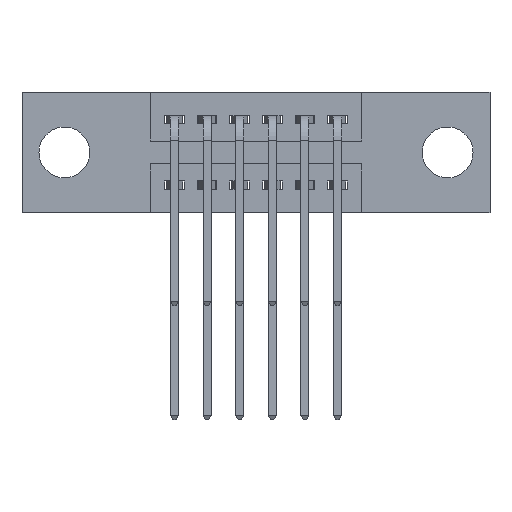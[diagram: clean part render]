
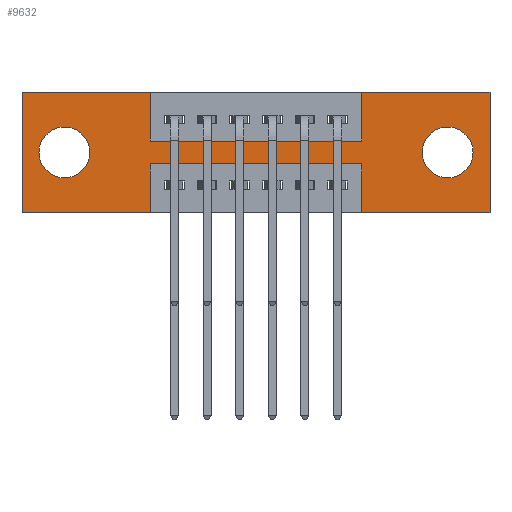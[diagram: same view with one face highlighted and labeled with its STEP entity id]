
A CAD part, front view. The second image highlights one B-rep face of the part: STEP entity #9632.
In plain terms, the highlighted planar face has unit normal (0, -1, 0).
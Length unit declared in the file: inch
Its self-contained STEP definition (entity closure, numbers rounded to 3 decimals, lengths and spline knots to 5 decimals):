
#202 = ORIENTED_EDGE ( 'NONE', *, *, #1817, .F. ) ;
#218 = EDGE_CURVE ( 'NONE', #5152, #11017, #5257, .T. ) ;
#248 = CARTESIAN_POINT ( 'NONE',  ( 1.435, 0., 0. ) ) ;
#366 = CARTESIAN_POINT ( 'NONE',  ( 1.0425, 0., 0. ) ) ;
#375 = ORIENTED_EDGE ( 'NONE', *, *, #869, .T. ) ;
#448 = ORIENTED_EDGE ( 'NONE', *, *, #2255, .F. ) ;
#457 = EDGE_LOOP ( 'NONE', ( #3153, #2119 ) ) ;
#676 = EDGE_CURVE ( 'NONE', #10058, #1149, #5128, .T. ) ;
#679 = CARTESIAN_POINT ( 'NONE',  ( 0.3925, 0., -0.15 ) ) ;
#805 = ORIENTED_EDGE ( 'NONE', *, *, #6886, .F. ) ;
#841 = ORIENTED_EDGE ( 'NONE', *, *, #6169, .F. ) ;
#858 = DIRECTION ( 'NONE',  ( -1., 0., 0. ) ) ;
#869 = EDGE_CURVE ( 'NONE', #1914, #2391, #6327, .T. ) ;
#880 = VECTOR ( 'NONE', #5306, 39.37008 ) ;
#924 = VERTEX_POINT ( 'NONE', #3868 ) ;
#1019 = LINE ( 'NONE', #8200, #11614 ) ;
#1138 = ORIENTED_EDGE ( 'NONE', *, *, #5997, .F. ) ;
#1149 = VERTEX_POINT ( 'NONE', #3234 ) ;
#1215 = ORIENTED_EDGE ( 'NONE', *, *, #7452, .F. ) ;
#1362 = CARTESIAN_POINT ( 'NONE',  ( 1.435, 0., 0. ) ) ;
#1496 = VERTEX_POINT ( 'NONE', #3971 ) ;
#1576 = ORIENTED_EDGE ( 'NONE', *, *, #4778, .F. ) ;
#1715 = CARTESIAN_POINT ( 'NONE',  ( 1.0425, 0., -0.22 ) ) ;
#1799 = VECTOR ( 'NONE', #5398, 39.37008 ) ;
#1817 = EDGE_CURVE ( 'NONE', #924, #9367, #1964, .T. ) ;
#1914 = VERTEX_POINT ( 'NONE', #6949 ) ;
#1964 = LINE ( 'NONE', #2258, #8264 ) ;
#2119 = ORIENTED_EDGE ( 'NONE', *, *, #8929, .T. ) ;
#2194 = CIRCLE ( 'NONE', #8778, 0.078 ) ;
#2255 = EDGE_CURVE ( 'NONE', #11017, #3963, #10328, .T. ) ;
#2258 = CARTESIAN_POINT ( 'NONE',  ( 0., 0., 0. ) ) ;
#2391 = VERTEX_POINT ( 'NONE', #8773 ) ;
#2502 = DIRECTION ( 'NONE',  ( 0., 0., -1. ) ) ;
#2565 = DIRECTION ( 'NONE',  ( 0., 0., -1. ) ) ;
#2607 = CARTESIAN_POINT ( 'NONE',  ( 1.0425, 0., 0. ) ) ;
#3078 = EDGE_LOOP ( 'NONE', ( #1576, #1138, #841, #6036, #448, #5516, #805, #4477, #9715, #202, #1215, #4601 ) ) ;
#3096 = DIRECTION ( 'NONE',  ( 0., 0., 1. ) ) ;
#3153 = ORIENTED_EDGE ( 'NONE', *, *, #5765, .T. ) ;
#3234 = CARTESIAN_POINT ( 'NONE',  ( 0., 0., -0.37 ) ) ;
#3313 = EDGE_LOOP ( 'NONE', ( #375, #4487 ) ) ;
#3424 = LINE ( 'NONE', #10508, #880 ) ;
#3464 = AXIS2_PLACEMENT_3D ( 'NONE', #5206, #7799, #11404 ) ;
#3525 = DIRECTION ( 'NONE',  ( 0., 0., 1. ) ) ;
#3554 = CARTESIAN_POINT ( 'NONE',  ( 0.13, 0., -0.107 ) ) ;
#3661 = VECTOR ( 'NONE', #7742, 39.37008 ) ;
#3772 = DIRECTION ( 'NONE',  ( 0., 0., 1. ) ) ;
#3849 = VECTOR ( 'NONE', #5325, 39.37008 ) ;
#3868 = CARTESIAN_POINT ( 'NONE',  ( 0., 0., 0. ) ) ;
#3963 = VERTEX_POINT ( 'NONE', #11116 ) ;
#3971 = CARTESIAN_POINT ( 'NONE',  ( 0.13, 0., -0.263 ) ) ;
#4007 = VECTOR ( 'NONE', #7783, 39.37008 ) ;
#4046 = VECTOR ( 'NONE', #4680, 39.37008 ) ;
#4062 = DIRECTION ( 'NONE',  ( 0., 0., 1. ) ) ;
#4194 = FACE_BOUND ( 'NONE', #457, .T. ) ;
#4234 = AXIS2_PLACEMENT_3D ( 'NONE', #6861, #5048, #3096 ) ;
#4254 = PLANE ( 'NONE',  #3464 ) ;
#4477 = ORIENTED_EDGE ( 'NONE', *, *, #9099, .F. ) ;
#4487 = ORIENTED_EDGE ( 'NONE', *, *, #6104, .T. ) ;
#4601 = ORIENTED_EDGE ( 'NONE', *, *, #676, .F. ) ;
#4642 = CARTESIAN_POINT ( 'NONE',  ( 1.305, 0., -0.185 ) ) ;
#4680 = DIRECTION ( 'NONE',  ( -1., 0., 0. ) ) ;
#4729 = DIRECTION ( 'NONE',  ( 0., 1., 0. ) ) ;
#4734 = LINE ( 'NONE', #5684, #4046 ) ;
#4778 = EDGE_CURVE ( 'NONE', #5113, #10058, #9640, .T. ) ;
#4889 = VECTOR ( 'NONE', #11262, 39.37008 ) ;
#5048 = DIRECTION ( 'NONE',  ( 0., 1., 0. ) ) ;
#5113 = VERTEX_POINT ( 'NONE', #7904 ) ;
#5128 = LINE ( 'NONE', #5892, #4007 ) ;
#5146 = CARTESIAN_POINT ( 'NONE',  ( 0.3925, 0., -0.37 ) ) ;
#5152 = VERTEX_POINT ( 'NONE', #2607 ) ;
#5206 = CARTESIAN_POINT ( 'NONE',  ( 0., 0., -0.37 ) ) ;
#5208 = VECTOR ( 'NONE', #4062, 39.37008 ) ;
#5257 = LINE ( 'NONE', #11345, #3661 ) ;
#5297 = DIRECTION ( 'NONE',  ( 0., 1., 0. ) ) ;
#5306 = DIRECTION ( 'NONE',  ( 0., 0., -1. ) ) ;
#5325 = DIRECTION ( 'NONE',  ( 1., 0., 0. ) ) ;
#5398 = DIRECTION ( 'NONE',  ( 0., 0., 1. ) ) ;
#5516 = ORIENTED_EDGE ( 'NONE', *, *, #218, .F. ) ;
#5606 = VERTEX_POINT ( 'NONE', #11378 ) ;
#5684 = CARTESIAN_POINT ( 'NONE',  ( 0., 0., -0.37 ) ) ;
#5765 = EDGE_CURVE ( 'NONE', #7993, #1496, #5954, .T. ) ;
#5892 = CARTESIAN_POINT ( 'NONE',  ( 0., 0., -0.37 ) ) ;
#5954 = CIRCLE ( 'NONE', #6139, 0.078 ) ;
#5997 = EDGE_CURVE ( 'NONE', #11311, #5113, #11640, .T. ) ;
#6036 = ORIENTED_EDGE ( 'NONE', *, *, #8811, .F. ) ;
#6104 = EDGE_CURVE ( 'NONE', #2391, #1914, #2194, .T. ) ;
#6139 = AXIS2_PLACEMENT_3D ( 'NONE', #9226, #4729, #3525 ) ;
#6144 = FACE_BOUND ( 'NONE', #3313, .T. ) ;
#6169 = EDGE_CURVE ( 'NONE', #8464, #11311, #1019, .T. ) ;
#6327 = CIRCLE ( 'NONE', #8397, 0.078 ) ;
#6491 = EDGE_CURVE ( 'NONE', #9367, #8373, #3424, .T. ) ;
#6861 = CARTESIAN_POINT ( 'NONE',  ( 0.13, 0., -0.185 ) ) ;
#6886 = EDGE_CURVE ( 'NONE', #5606, #5152, #9314, .T. ) ;
#6910 = FACE_OUTER_BOUND ( 'NONE', #3078, .T. ) ;
#6949 = CARTESIAN_POINT ( 'NONE',  ( 1.305, 0., -0.107 ) ) ;
#7278 = CARTESIAN_POINT ( 'NONE',  ( 0., 0., 0. ) ) ;
#7452 = EDGE_CURVE ( 'NONE', #1149, #924, #10002, .T. ) ;
#7742 = DIRECTION ( 'NONE',  ( 1., 0., 0. ) ) ;
#7783 = DIRECTION ( 'NONE',  ( -1., 0., 0. ) ) ;
#7799 = DIRECTION ( 'NONE',  ( 0., -1., 0. ) ) ;
#7904 = CARTESIAN_POINT ( 'NONE',  ( 0.3925, 0., -0.22 ) ) ;
#7993 = VERTEX_POINT ( 'NONE', #3554 ) ;
#8200 = CARTESIAN_POINT ( 'NONE',  ( 1.0425, 0., -0.37 ) ) ;
#8237 = DIRECTION ( 'NONE',  ( 0., 0., -1. ) ) ;
#8264 = VECTOR ( 'NONE', #11274, 39.37008 ) ;
#8373 = VERTEX_POINT ( 'NONE', #679 ) ;
#8397 = AXIS2_PLACEMENT_3D ( 'NONE', #4642, #5297, #8237 ) ;
#8464 = VERTEX_POINT ( 'NONE', #8904 ) ;
#8751 = CARTESIAN_POINT ( 'NONE',  ( 0.3925, 0., -0.15 ) ) ;
#8773 = CARTESIAN_POINT ( 'NONE',  ( 1.305, 0., -0.263 ) ) ;
#8778 = AXIS2_PLACEMENT_3D ( 'NONE', #9819, #11522, #2565 ) ;
#8811 = EDGE_CURVE ( 'NONE', #3963, #8464, #4734, .T. ) ;
#8904 = CARTESIAN_POINT ( 'NONE',  ( 1.0425, 0., -0.37 ) ) ;
#8929 = EDGE_CURVE ( 'NONE', #1496, #7993, #11218, .T. ) ;
#9099 = EDGE_CURVE ( 'NONE', #8373, #5606, #9590, .T. ) ;
#9226 = CARTESIAN_POINT ( 'NONE',  ( 0.13, 0., -0.185 ) ) ;
#9314 = LINE ( 'NONE', #366, #5208 ) ;
#9326 = VECTOR ( 'NONE', #2502, 39.37008 ) ;
#9367 = VERTEX_POINT ( 'NONE', #10804 ) ;
#9590 = LINE ( 'NONE', #8751, #3849 ) ;
#9632 = ADVANCED_FACE ( 'NONE', ( #6144, #4194, #6910 ), #4254, .T. ) ;
#9640 = LINE ( 'NONE', #5146, #9326 ) ;
#9644 = CARTESIAN_POINT ( 'NONE',  ( 0.3925, 0., -0.22 ) ) ;
#9715 = ORIENTED_EDGE ( 'NONE', *, *, #6491, .F. ) ;
#9819 = CARTESIAN_POINT ( 'NONE',  ( 1.305, 0., -0.185 ) ) ;
#10002 = LINE ( 'NONE', #7278, #1799 ) ;
#10058 = VERTEX_POINT ( 'NONE', #10439 ) ;
#10328 = LINE ( 'NONE', #1362, #4889 ) ;
#10439 = CARTESIAN_POINT ( 'NONE',  ( 0.3925, 0., -0.37 ) ) ;
#10508 = CARTESIAN_POINT ( 'NONE',  ( 0.3925, 0., 0. ) ) ;
#10804 = CARTESIAN_POINT ( 'NONE',  ( 0.3925, 0., 0. ) ) ;
#11017 = VERTEX_POINT ( 'NONE', #248 ) ;
#11116 = CARTESIAN_POINT ( 'NONE',  ( 1.435, 0., -0.37 ) ) ;
#11218 = CIRCLE ( 'NONE', #4234, 0.078 ) ;
#11262 = DIRECTION ( 'NONE',  ( 0., 0., -1. ) ) ;
#11274 = DIRECTION ( 'NONE',  ( 1., 0., 0. ) ) ;
#11311 = VERTEX_POINT ( 'NONE', #1715 ) ;
#11345 = CARTESIAN_POINT ( 'NONE',  ( 0., 0., 0. ) ) ;
#11378 = CARTESIAN_POINT ( 'NONE',  ( 1.0425, 0., -0.15 ) ) ;
#11404 = DIRECTION ( 'NONE',  ( 0., 0., -1. ) ) ;
#11422 = VECTOR ( 'NONE', #858, 39.37008 ) ;
#11522 = DIRECTION ( 'NONE',  ( 0., 1., 0. ) ) ;
#11614 = VECTOR ( 'NONE', #3772, 39.37008 ) ;
#11640 = LINE ( 'NONE', #9644, #11422 ) ;
